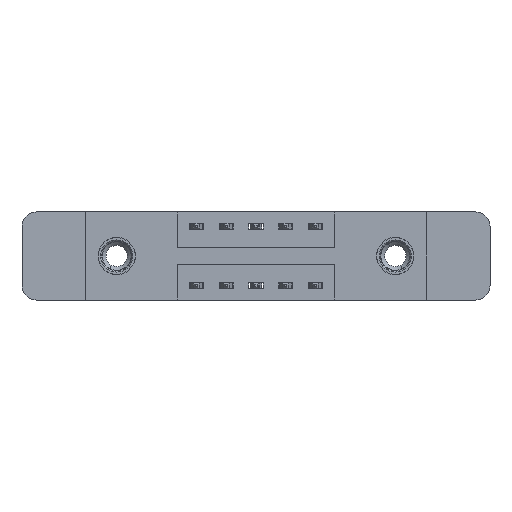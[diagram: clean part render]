
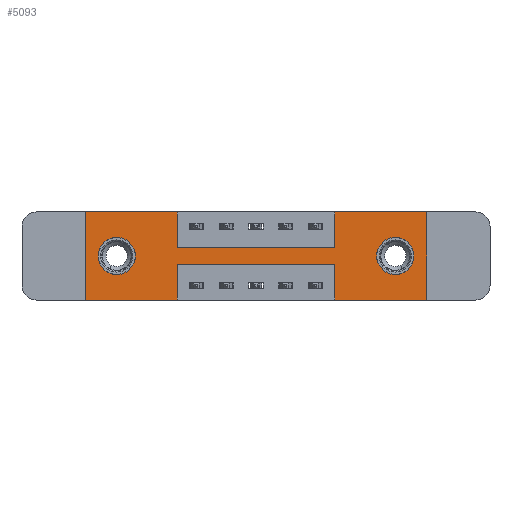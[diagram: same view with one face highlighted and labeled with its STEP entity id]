
A CAD part, front view. The second image highlights one B-rep face of the part: STEP entity #5093.
In plain terms, the highlighted planar face has unit normal (0, -1, 0).
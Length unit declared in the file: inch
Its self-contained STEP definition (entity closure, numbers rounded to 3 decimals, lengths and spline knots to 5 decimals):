
#83 = ORIENTED_EDGE ( 'NONE', *, *, #3836, .F. ) ;
#120 = VECTOR ( 'NONE', #2317, 39.37008 ) ;
#258 = CARTESIAN_POINT ( 'NONE',  ( 0., 0., 0. ) ) ;
#310 = VECTOR ( 'NONE', #9584, 39.37008 ) ;
#322 = CARTESIAN_POINT ( 'NONE',  ( 1.0475, 0., -0.37 ) ) ;
#323 = ORIENTED_EDGE ( 'NONE', *, *, #10446, .T. ) ;
#676 = CARTESIAN_POINT ( 'NONE',  ( 0.3875, 0., 0. ) ) ;
#725 = LINE ( 'NONE', #10286, #5495 ) ;
#747 = LINE ( 'NONE', #7219, #4375 ) ;
#810 = DIRECTION ( 'NONE',  ( 0., 0., -1. ) ) ;
#827 = EDGE_CURVE ( 'NONE', #9300, #4303, #9181, .T. ) ;
#913 = ORIENTED_EDGE ( 'NONE', *, *, #7228, .F. ) ;
#1005 = DIRECTION ( 'NONE',  ( 0., 1., 0. ) ) ;
#1082 = CARTESIAN_POINT ( 'NONE',  ( 0., 0., -0.37 ) ) ;
#1118 = VERTEX_POINT ( 'NONE', #2353 ) ;
#1303 = DIRECTION ( 'NONE',  ( -1., 0., 0. ) ) ;
#1597 = LINE ( 'NONE', #2793, #5214 ) ;
#1714 = CARTESIAN_POINT ( 'NONE',  ( 0.3875, 0., -0.37 ) ) ;
#1745 = ORIENTED_EDGE ( 'NONE', *, *, #2524, .F. ) ;
#1791 = VECTOR ( 'NONE', #2709, 39.37008 ) ;
#1835 = VERTEX_POINT ( 'NONE', #7158 ) ;
#2317 = DIRECTION ( 'NONE',  ( 0., 0., 1. ) ) ;
#2334 = CARTESIAN_POINT ( 'NONE',  ( 1.0475, 0., 0. ) ) ;
#2353 = CARTESIAN_POINT ( 'NONE',  ( 1.435, 0., 0. ) ) ;
#2501 = LINE ( 'NONE', #1714, #11029 ) ;
#2524 = EDGE_CURVE ( 'NONE', #6871, #4920, #10914, .T. ) ;
#2709 = DIRECTION ( 'NONE',  ( 1., 0., 0. ) ) ;
#2793 = CARTESIAN_POINT ( 'NONE',  ( 0.3875, 0., -0.22 ) ) ;
#2855 = EDGE_LOOP ( 'NONE', ( #10621, #5381, #8355, #1745, #4212, #7856, #913, #83, #4102, #6574, #7015, #4234 ) ) ;
#2914 = EDGE_LOOP ( 'NONE', ( #7880, #13377 ) ) ;
#3074 = DIRECTION ( 'NONE',  ( -1., 0., 0. ) ) ;
#3227 = VECTOR ( 'NONE', #1303, 39.37008 ) ;
#3284 = VERTEX_POINT ( 'NONE', #12322 ) ;
#3464 = VERTEX_POINT ( 'NONE', #12598 ) ;
#3609 = DIRECTION ( 'NONE',  ( 0., 1., 0. ) ) ;
#3664 = CARTESIAN_POINT ( 'NONE',  ( 0.3875, 0., 0. ) ) ;
#3736 = EDGE_CURVE ( 'NONE', #3464, #13471, #2501, .T. ) ;
#3836 = EDGE_CURVE ( 'NONE', #4303, #5869, #12307, .T. ) ;
#3880 = CARTESIAN_POINT ( 'NONE',  ( 1.0475, 0., -0.15 ) ) ;
#4043 = CARTESIAN_POINT ( 'NONE',  ( 0.1325, 0., -0.263 ) ) ;
#4102 = ORIENTED_EDGE ( 'NONE', *, *, #827, .F. ) ;
#4157 = VECTOR ( 'NONE', #6996, 39.37008 ) ;
#4185 = AXIS2_PLACEMENT_3D ( 'NONE', #9191, #12336, #8071 ) ;
#4211 = AXIS2_PLACEMENT_3D ( 'NONE', #7473, #1005, #12956 ) ;
#4212 = ORIENTED_EDGE ( 'NONE', *, *, #7707, .F. ) ;
#4234 = ORIENTED_EDGE ( 'NONE', *, *, #10293, .F. ) ;
#4303 = VERTEX_POINT ( 'NONE', #11100 ) ;
#4375 = VECTOR ( 'NONE', #3074, 39.37008 ) ;
#4556 = LINE ( 'NONE', #5675, #120 ) ;
#4808 = FACE_BOUND ( 'NONE', #2914, .T. ) ;
#4879 = CIRCLE ( 'NONE', #4211, 0.078 ) ;
#4920 = VERTEX_POINT ( 'NONE', #322 ) ;
#5016 = FACE_OUTER_BOUND ( 'NONE', #2855, .T. ) ;
#5093 = ADVANCED_FACE ( 'NONE', ( #13525, #4808, #5016 ), #7218, .T. ) ;
#5214 = VECTOR ( 'NONE', #5864, 39.37008 ) ;
#5381 = ORIENTED_EDGE ( 'NONE', *, *, #6500, .F. ) ;
#5495 = VECTOR ( 'NONE', #13578, 39.37008 ) ;
#5511 = CARTESIAN_POINT ( 'NONE',  ( 1.435, 0., -0.37 ) ) ;
#5588 = EDGE_CURVE ( 'NONE', #13484, #1835, #4879, .T. ) ;
#5675 = CARTESIAN_POINT ( 'NONE',  ( 1.0475, 0., -0.37 ) ) ;
#5864 = DIRECTION ( 'NONE',  ( -1., 0., 0. ) ) ;
#5869 = VERTEX_POINT ( 'NONE', #3880 ) ;
#6186 = VERTEX_POINT ( 'NONE', #11552 ) ;
#6329 = LINE ( 'NONE', #10617, #310 ) ;
#6397 = EDGE_CURVE ( 'NONE', #9018, #1118, #7985, .T. ) ;
#6439 = VERTEX_POINT ( 'NONE', #4043 ) ;
#6500 = EDGE_CURVE ( 'NONE', #8497, #3464, #1597, .T. ) ;
#6501 = CARTESIAN_POINT ( 'NONE',  ( 1.3025, 0., -0.185 ) ) ;
#6574 = ORIENTED_EDGE ( 'NONE', *, *, #7194, .F. ) ;
#6579 = DIRECTION ( 'NONE',  ( 1., 0., 0. ) ) ;
#6740 = AXIS2_PLACEMENT_3D ( 'NONE', #9318, #12395, #7001 ) ;
#6871 = VERTEX_POINT ( 'NONE', #5511 ) ;
#6996 = DIRECTION ( 'NONE',  ( 0., 0., -1. ) ) ;
#7001 = DIRECTION ( 'NONE',  ( 0., 0., -1. ) ) ;
#7015 = ORIENTED_EDGE ( 'NONE', *, *, #8045, .F. ) ;
#7158 = CARTESIAN_POINT ( 'NONE',  ( 1.3025, 0., -0.263 ) ) ;
#7194 = EDGE_CURVE ( 'NONE', #6186, #9300, #6329, .T. ) ;
#7218 = PLANE ( 'NONE',  #6740 ) ;
#7219 = CARTESIAN_POINT ( 'NONE',  ( 0., 0., -0.37 ) ) ;
#7228 = EDGE_CURVE ( 'NONE', #5869, #9018, #8661, .T. ) ;
#7473 = CARTESIAN_POINT ( 'NONE',  ( 1.3025, 0., -0.185 ) ) ;
#7707 = EDGE_CURVE ( 'NONE', #1118, #6871, #12465, .T. ) ;
#7791 = AXIS2_PLACEMENT_3D ( 'NONE', #6501, #8605, #12886 ) ;
#7827 = DIRECTION ( 'NONE',  ( 0., 0., 1. ) ) ;
#7856 = ORIENTED_EDGE ( 'NONE', *, *, #6397, .F. ) ;
#7880 = ORIENTED_EDGE ( 'NONE', *, *, #8293, .T. ) ;
#7985 = LINE ( 'NONE', #258, #9056 ) ;
#8045 = EDGE_CURVE ( 'NONE', #12378, #6186, #725, .T. ) ;
#8071 = DIRECTION ( 'NONE',  ( 0., 0., 1. ) ) ;
#8110 = CARTESIAN_POINT ( 'NONE',  ( 0.3875, 0., -0.15 ) ) ;
#8293 = EDGE_CURVE ( 'NONE', #3284, #6439, #11751, .T. ) ;
#8305 = CARTESIAN_POINT ( 'NONE',  ( 0., 0., -0.37 ) ) ;
#8355 = ORIENTED_EDGE ( 'NONE', *, *, #8668, .F. ) ;
#8497 = VERTEX_POINT ( 'NONE', #13279 ) ;
#8605 = DIRECTION ( 'NONE',  ( 0., 1., 0. ) ) ;
#8661 = LINE ( 'NONE', #2334, #12188 ) ;
#8668 = EDGE_CURVE ( 'NONE', #4920, #8497, #4556, .T. ) ;
#9018 = VERTEX_POINT ( 'NONE', #13685 ) ;
#9021 = DIRECTION ( 'NONE',  ( 0., 0., -1. ) ) ;
#9056 = VECTOR ( 'NONE', #6579, 39.37008 ) ;
#9181 = LINE ( 'NONE', #676, #4157 ) ;
#9191 = CARTESIAN_POINT ( 'NONE',  ( 0.1325, 0., -0.185 ) ) ;
#9300 = VERTEX_POINT ( 'NONE', #3664 ) ;
#9318 = CARTESIAN_POINT ( 'NONE',  ( 0., 0., -0.37 ) ) ;
#9584 = DIRECTION ( 'NONE',  ( 1., 0., 0. ) ) ;
#9933 = CARTESIAN_POINT ( 'NONE',  ( 0.1325, 0., -0.185 ) ) ;
#10286 = CARTESIAN_POINT ( 'NONE',  ( 0., 0., 0. ) ) ;
#10293 = EDGE_CURVE ( 'NONE', #13471, #12378, #747, .T. ) ;
#10435 = CARTESIAN_POINT ( 'NONE',  ( 1.435, 0., 0. ) ) ;
#10446 = EDGE_CURVE ( 'NONE', #1835, #13484, #13819, .T. ) ;
#10617 = CARTESIAN_POINT ( 'NONE',  ( 0., 0., 0. ) ) ;
#10621 = ORIENTED_EDGE ( 'NONE', *, *, #3736, .F. ) ;
#10697 = CIRCLE ( 'NONE', #4185, 0.078 ) ;
#10914 = LINE ( 'NONE', #1082, #3227 ) ;
#11029 = VECTOR ( 'NONE', #9021, 39.37008 ) ;
#11100 = CARTESIAN_POINT ( 'NONE',  ( 0.3875, 0., -0.15 ) ) ;
#11552 = CARTESIAN_POINT ( 'NONE',  ( 0., 0., 0. ) ) ;
#11751 = CIRCLE ( 'NONE', #12204, 0.078 ) ;
#11832 = EDGE_LOOP ( 'NONE', ( #12290, #323 ) ) ;
#12148 = DIRECTION ( 'NONE',  ( 0., 0., 1. ) ) ;
#12188 = VECTOR ( 'NONE', #12148, 39.37008 ) ;
#12204 = AXIS2_PLACEMENT_3D ( 'NONE', #9933, #3609, #7827 ) ;
#12290 = ORIENTED_EDGE ( 'NONE', *, *, #5588, .T. ) ;
#12307 = LINE ( 'NONE', #8110, #1791 ) ;
#12322 = CARTESIAN_POINT ( 'NONE',  ( 0.1325, 0., -0.107 ) ) ;
#12336 = DIRECTION ( 'NONE',  ( 0., 1., 0. ) ) ;
#12378 = VERTEX_POINT ( 'NONE', #8305 ) ;
#12395 = DIRECTION ( 'NONE',  ( 0., -1., 0. ) ) ;
#12465 = LINE ( 'NONE', #10435, #13108 ) ;
#12598 = CARTESIAN_POINT ( 'NONE',  ( 0.3875, 0., -0.22 ) ) ;
#12657 = EDGE_CURVE ( 'NONE', #6439, #3284, #10697, .T. ) ;
#12886 = DIRECTION ( 'NONE',  ( 0., 0., -1. ) ) ;
#12956 = DIRECTION ( 'NONE',  ( 0., 0., -1. ) ) ;
#13108 = VECTOR ( 'NONE', #810, 39.37008 ) ;
#13222 = CARTESIAN_POINT ( 'NONE',  ( 0.3875, 0., -0.37 ) ) ;
#13279 = CARTESIAN_POINT ( 'NONE',  ( 1.0475, 0., -0.22 ) ) ;
#13377 = ORIENTED_EDGE ( 'NONE', *, *, #12657, .T. ) ;
#13471 = VERTEX_POINT ( 'NONE', #13222 ) ;
#13484 = VERTEX_POINT ( 'NONE', #13495 ) ;
#13495 = CARTESIAN_POINT ( 'NONE',  ( 1.3025, 0., -0.107 ) ) ;
#13525 = FACE_BOUND ( 'NONE', #11832, .T. ) ;
#13578 = DIRECTION ( 'NONE',  ( 0., 0., 1. ) ) ;
#13685 = CARTESIAN_POINT ( 'NONE',  ( 1.0475, 0., 0. ) ) ;
#13819 = CIRCLE ( 'NONE', #7791, 0.078 ) ;
